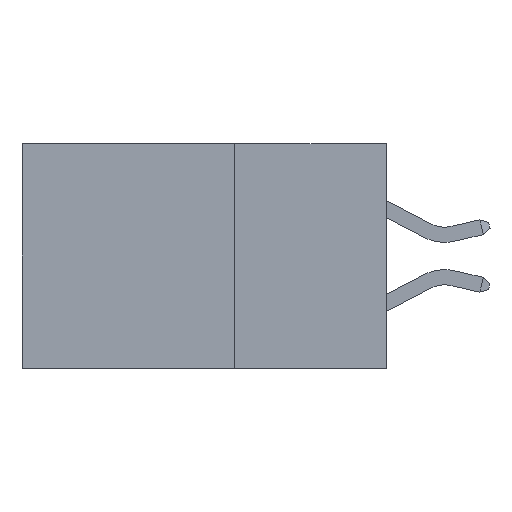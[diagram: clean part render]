
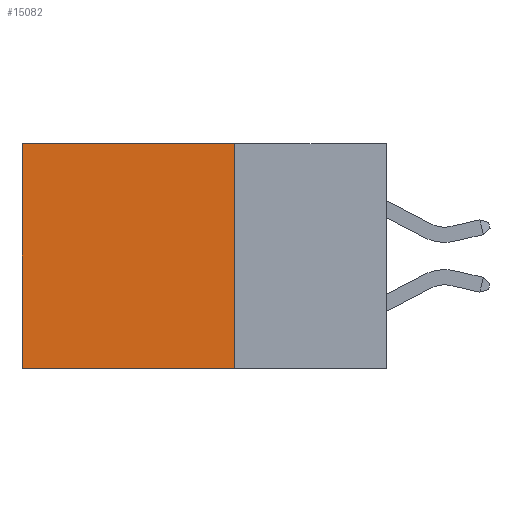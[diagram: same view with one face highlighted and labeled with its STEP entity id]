
A CAD part, left-side view. The second image highlights one B-rep face of the part: STEP entity #15082.
In plain terms, the highlighted planar face has unit normal (-1, 0, 0).
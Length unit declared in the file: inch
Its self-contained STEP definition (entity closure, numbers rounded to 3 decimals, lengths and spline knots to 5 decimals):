
#822 = VERTEX_POINT ( 'NONE', #13601 ) ;
#832 = EDGE_CURVE ( 'NONE', #822, #10746, #23039, .T. ) ;
#1745 = EDGE_LOOP ( 'NONE', ( #2385, #2447, #11696, #24519 ) ) ;
#1894 = PLANE ( 'NONE',  #3235 ) ;
#2385 = ORIENTED_EDGE ( 'NONE', *, *, #11883, .T. ) ;
#2447 = ORIENTED_EDGE ( 'NONE', *, *, #832, .F. ) ;
#2810 = DIRECTION ( 'NONE',  ( 0., 1., 0. ) ) ;
#3235 = AXIS2_PLACEMENT_3D ( 'NONE', #23063, #3869, #17568 ) ;
#3382 = CARTESIAN_POINT ( 'NONE',  ( 0.298, 0.25, 0. ) ) ;
#3869 = DIRECTION ( 'NONE',  ( 1., 0., 0. ) ) ;
#4740 = LINE ( 'NONE', #11083, #8732 ) ;
#6222 = CARTESIAN_POINT ( 'NONE',  ( 0.298, 0.25, 0. ) ) ;
#6926 = VECTOR ( 'NONE', #2810, 39.37008 ) ;
#7643 = VECTOR ( 'NONE', #14103, 39.37008 ) ;
#8582 = LINE ( 'NONE', #6222, #13210 ) ;
#8732 = VECTOR ( 'NONE', #13059, 39.37008 ) ;
#10563 = VERTEX_POINT ( 'NONE', #3382 ) ;
#10606 = VERTEX_POINT ( 'NONE', #24703 ) ;
#10746 = VERTEX_POINT ( 'NONE', #15686 ) ;
#11083 = CARTESIAN_POINT ( 'NONE',  ( 0.298, 0.6, 0. ) ) ;
#11696 = ORIENTED_EDGE ( 'NONE', *, *, #21198, .F. ) ;
#11883 = EDGE_CURVE ( 'NONE', #10606, #10746, #4740, .T. ) ;
#12177 = DIRECTION ( 'NONE',  ( 0., 0., -1. ) ) ;
#12793 = CARTESIAN_POINT ( 'NONE',  ( 0.298, 0.25, -0.37 ) ) ;
#13059 = DIRECTION ( 'NONE',  ( 0., 0., -1. ) ) ;
#13210 = VECTOR ( 'NONE', #12177, 39.37008 ) ;
#13601 = CARTESIAN_POINT ( 'NONE',  ( 0.298, 0.25, -0.37 ) ) ;
#14103 = DIRECTION ( 'NONE',  ( 0., 1., 0. ) ) ;
#15082 = ADVANCED_FACE ( 'NONE', ( #19656 ), #1894, .F. ) ;
#15686 = CARTESIAN_POINT ( 'NONE',  ( 0.298, 0.6, -0.37 ) ) ;
#16553 = CARTESIAN_POINT ( 'NONE',  ( 0.298, 0.25, 0. ) ) ;
#17568 = DIRECTION ( 'NONE',  ( 0., 0., -1. ) ) ;
#19656 = FACE_OUTER_BOUND ( 'NONE', #1745, .T. ) ;
#21198 = EDGE_CURVE ( 'NONE', #10563, #822, #8582, .T. ) ;
#21744 = LINE ( 'NONE', #16553, #6926 ) ;
#23039 = LINE ( 'NONE', #12793, #7643 ) ;
#23063 = CARTESIAN_POINT ( 'NONE',  ( 0.298, 0.25, 0. ) ) ;
#23667 = EDGE_CURVE ( 'NONE', #10563, #10606, #21744, .T. ) ;
#24519 = ORIENTED_EDGE ( 'NONE', *, *, #23667, .T. ) ;
#24703 = CARTESIAN_POINT ( 'NONE',  ( 0.298, 0.6, 0. ) ) ;
